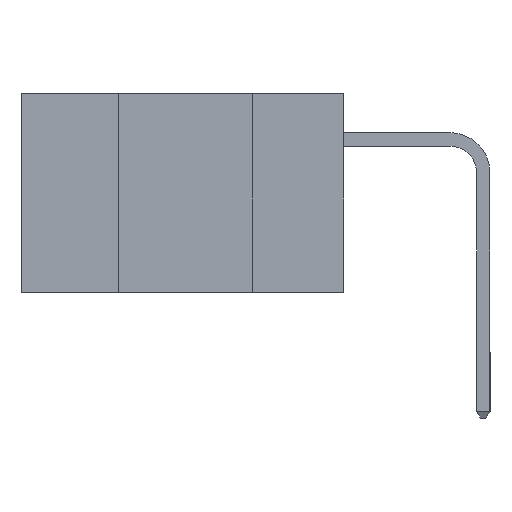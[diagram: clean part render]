
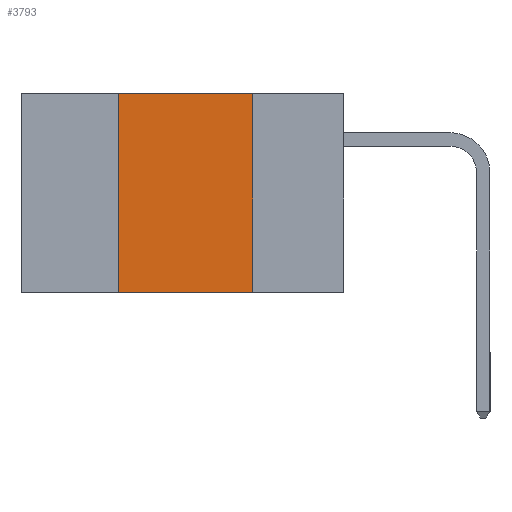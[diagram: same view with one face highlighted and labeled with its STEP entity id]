
A CAD part, left-side view. The second image highlights one B-rep face of the part: STEP entity #3793.
In plain terms, the highlighted planar face has unit normal (-1, 0, 0).
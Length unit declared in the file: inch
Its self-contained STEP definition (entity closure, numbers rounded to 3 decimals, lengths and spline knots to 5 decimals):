
#838 = VECTOR ( 'NONE', #2097, 39.37008 ) ;
#870 = ORIENTED_EDGE ( 'NONE', *, *, #1357, .F. ) ;
#1328 = EDGE_CURVE ( 'NONE', #12061, #14115, #14446, .T. ) ;
#1357 = EDGE_CURVE ( 'NONE', #14115, #15429, #7709, .T. ) ;
#1749 = CARTESIAN_POINT ( 'NONE',  ( 0., 0.6, 0. ) ) ;
#2087 = DIRECTION ( 'NONE',  ( 1., 0., 0. ) ) ;
#2097 = DIRECTION ( 'NONE',  ( 0., -1., 0. ) ) ;
#2336 = CARTESIAN_POINT ( 'NONE',  ( 0., 0.17, 0. ) ) ;
#3471 = FACE_OUTER_BOUND ( 'NONE', #13693, .T. ) ;
#3793 = ADVANCED_FACE ( 'NONE', ( #3471 ), #17454, .F. ) ;
#4195 = LINE ( 'NONE', #16895, #13720 ) ;
#4285 = CARTESIAN_POINT ( 'NONE',  ( 0., 0.42, 0. ) ) ;
#4870 = CARTESIAN_POINT ( 'NONE',  ( 0., 0.6, 0. ) ) ;
#4980 = AXIS2_PLACEMENT_3D ( 'NONE', #4870, #2087, #8816 ) ;
#6729 = CARTESIAN_POINT ( 'NONE',  ( 0., 0.42, -0.37 ) ) ;
#7080 = ORIENTED_EDGE ( 'NONE', *, *, #14741, .T. ) ;
#7314 = VECTOR ( 'NONE', #7440, 39.37008 ) ;
#7440 = DIRECTION ( 'NONE',  ( 0., 0., -1. ) ) ;
#7709 = LINE ( 'NONE', #13249, #7314 ) ;
#8250 = CARTESIAN_POINT ( 'NONE',  ( 0., 0.17, -0.37 ) ) ;
#8533 = CARTESIAN_POINT ( 'NONE',  ( 0., 0.42, -0.37 ) ) ;
#8816 = DIRECTION ( 'NONE',  ( 0., 0., -1. ) ) ;
#10000 = DIRECTION ( 'NONE',  ( 0., -1., 0. ) ) ;
#10492 = VECTOR ( 'NONE', #15431, 39.37008 ) ;
#11470 = ORIENTED_EDGE ( 'NONE', *, *, #1328, .F. ) ;
#12061 = VERTEX_POINT ( 'NONE', #4285 ) ;
#12767 = LINE ( 'NONE', #6729, #10492 ) ;
#12834 = ORIENTED_EDGE ( 'NONE', *, *, #14659, .F. ) ;
#13249 = CARTESIAN_POINT ( 'NONE',  ( 0., 0.17, -0.37 ) ) ;
#13693 = EDGE_LOOP ( 'NONE', ( #870, #11470, #12834, #7080 ) ) ;
#13720 = VECTOR ( 'NONE', #10000, 39.37008 ) ;
#14115 = VERTEX_POINT ( 'NONE', #2336 ) ;
#14446 = LINE ( 'NONE', #1749, #838 ) ;
#14659 = EDGE_CURVE ( 'NONE', #16912, #12061, #12767, .T. ) ;
#14741 = EDGE_CURVE ( 'NONE', #16912, #15429, #4195, .T. ) ;
#15429 = VERTEX_POINT ( 'NONE', #8250 ) ;
#15431 = DIRECTION ( 'NONE',  ( 0., 0., 1. ) ) ;
#16895 = CARTESIAN_POINT ( 'NONE',  ( 0., 0.6, -0.37 ) ) ;
#16912 = VERTEX_POINT ( 'NONE', #8533 ) ;
#17454 = PLANE ( 'NONE',  #4980 ) ;
